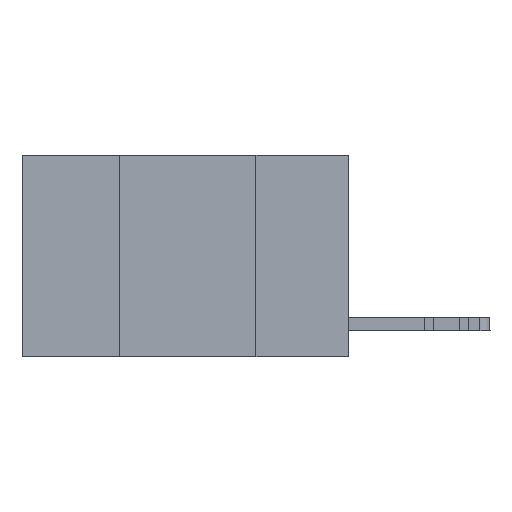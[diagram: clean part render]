
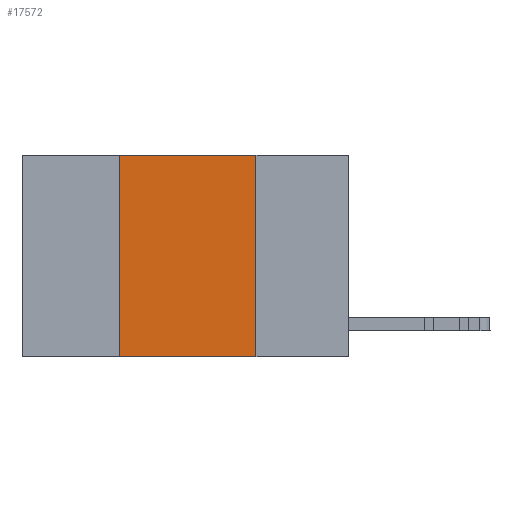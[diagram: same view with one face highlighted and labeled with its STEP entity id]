
A CAD part, left-side view. The second image highlights one B-rep face of the part: STEP entity #17572.
In plain terms, the highlighted planar face has unit normal (-1, 0, 0).
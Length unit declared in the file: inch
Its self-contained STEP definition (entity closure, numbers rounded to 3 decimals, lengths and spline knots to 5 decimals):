
#613 = VECTOR ( 'NONE', #25061, 39.37008 ) ;
#1010 = EDGE_LOOP ( 'NONE', ( #7454, #13329, #2989, #29881 ) ) ;
#1134 = EDGE_CURVE ( 'NONE', #11062, #25594, #4299, .T. ) ;
#1307 = CARTESIAN_POINT ( 'NONE',  ( 0., 0.6, 0. ) ) ;
#1816 = CARTESIAN_POINT ( 'NONE',  ( 0., 0.6, -0.37 ) ) ;
#1954 = LINE ( 'NONE', #20344, #16363 ) ;
#2989 = ORIENTED_EDGE ( 'NONE', *, *, #19353, .F. ) ;
#4299 = LINE ( 'NONE', #27084, #21525 ) ;
#6524 = CARTESIAN_POINT ( 'NONE',  ( 0., 0.17, -0.37 ) ) ;
#7454 = ORIENTED_EDGE ( 'NONE', *, *, #19430, .F. ) ;
#8054 = CARTESIAN_POINT ( 'NONE',  ( 0., 0.42, 0. ) ) ;
#8298 = DIRECTION ( 'NONE',  ( 0., 0., -1. ) ) ;
#9259 = LINE ( 'NONE', #1816, #613 ) ;
#10576 = DIRECTION ( 'NONE',  ( 1., 0., 0. ) ) ;
#11062 = VERTEX_POINT ( 'NONE', #28374 ) ;
#11223 = DIRECTION ( 'NONE',  ( 0., 0., -1. ) ) ;
#12944 = VERTEX_POINT ( 'NONE', #6524 ) ;
#13161 = PLANE ( 'NONE',  #16839 ) ;
#13329 = ORIENTED_EDGE ( 'NONE', *, *, #1134, .F. ) ;
#13563 = DIRECTION ( 'NONE',  ( 0., -1., 0. ) ) ;
#16363 = VECTOR ( 'NONE', #11223, 39.37008 ) ;
#16839 = AXIS2_PLACEMENT_3D ( 'NONE', #1307, #10576, #8298 ) ;
#17026 = LINE ( 'NONE', #8054, #18291 ) ;
#17572 = ADVANCED_FACE ( 'NONE', ( #29123 ), #13161, .F. ) ;
#18291 = VECTOR ( 'NONE', #29024, 39.37008 ) ;
#18356 = VERTEX_POINT ( 'NONE', #19779 ) ;
#19353 = EDGE_CURVE ( 'NONE', #18356, #11062, #17026, .T. ) ;
#19430 = EDGE_CURVE ( 'NONE', #25594, #12944, #1954, .T. ) ;
#19779 = CARTESIAN_POINT ( 'NONE',  ( 0., 0.42, -0.37 ) ) ;
#20344 = CARTESIAN_POINT ( 'NONE',  ( 0., 0.17, 0. ) ) ;
#21525 = VECTOR ( 'NONE', #13563, 39.37008 ) ;
#21995 = EDGE_CURVE ( 'NONE', #18356, #12944, #9259, .T. ) ;
#25061 = DIRECTION ( 'NONE',  ( 0., -1., 0. ) ) ;
#25594 = VERTEX_POINT ( 'NONE', #29790 ) ;
#27084 = CARTESIAN_POINT ( 'NONE',  ( 0., 0.6, 0. ) ) ;
#28374 = CARTESIAN_POINT ( 'NONE',  ( 0., 0.42, 0. ) ) ;
#29024 = DIRECTION ( 'NONE',  ( 0., 0., 1. ) ) ;
#29123 = FACE_OUTER_BOUND ( 'NONE', #1010, .T. ) ;
#29790 = CARTESIAN_POINT ( 'NONE',  ( 0., 0.17, 0. ) ) ;
#29881 = ORIENTED_EDGE ( 'NONE', *, *, #21995, .T. ) ;
